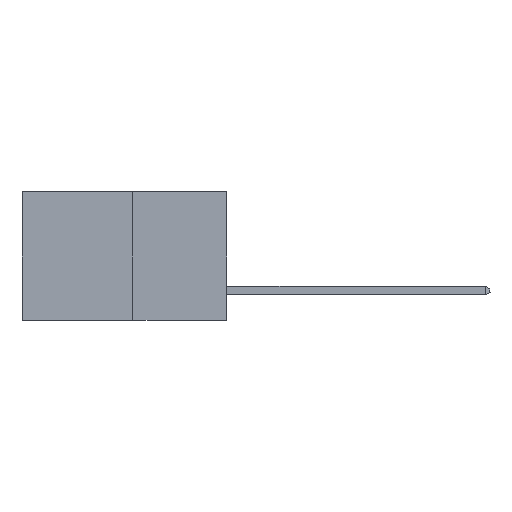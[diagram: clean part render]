
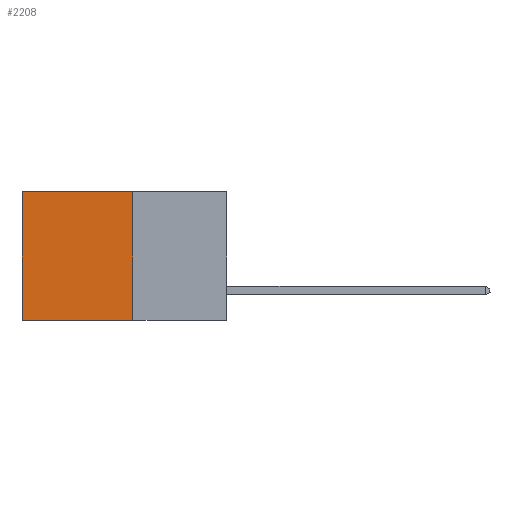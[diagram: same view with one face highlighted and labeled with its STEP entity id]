
A CAD part, left-side view. The second image highlights one B-rep face of the part: STEP entity #2208.
In plain terms, the highlighted planar face has unit normal (-1, 0, 0).
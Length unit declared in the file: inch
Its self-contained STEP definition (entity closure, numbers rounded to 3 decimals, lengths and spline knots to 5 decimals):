
#1157 = EDGE_CURVE ( 'NONE', #11840, #10073, #4215, .T. ) ;
#1207 = VECTOR ( 'NONE', #7720, 39.37008 ) ;
#1565 = EDGE_CURVE ( 'NONE', #10487, #11840, #7349, .T. ) ;
#2208 = ADVANCED_FACE ( 'NONE', ( #12992 ), #5448, .F. ) ;
#2436 = VECTOR ( 'NONE', #4837, 39.37008 ) ;
#4215 = LINE ( 'NONE', #14413, #1207 ) ;
#4347 = CARTESIAN_POINT ( 'NONE',  ( 0.277, 0.27, 0. ) ) ;
#4805 = CARTESIAN_POINT ( 'NONE',  ( 0.277, 0.27, -0.37 ) ) ;
#4837 = DIRECTION ( 'NONE',  ( 0., 1., 0. ) ) ;
#4951 = VECTOR ( 'NONE', #13122, 39.37008 ) ;
#5448 = PLANE ( 'NONE',  #10220 ) ;
#5536 = LINE ( 'NONE', #12847, #2436 ) ;
#5865 = VECTOR ( 'NONE', #13936, 39.37008 ) ;
#5984 = DIRECTION ( 'NONE',  ( 0., 0., -1. ) ) ;
#6015 = DIRECTION ( 'NONE',  ( 1., 0., 0. ) ) ;
#6047 = CARTESIAN_POINT ( 'NONE',  ( 0.277, 0.27, -0.37 ) ) ;
#6055 = VERTEX_POINT ( 'NONE', #6295 ) ;
#6295 = CARTESIAN_POINT ( 'NONE',  ( 0.277, 0.27, -0.37 ) ) ;
#7349 = LINE ( 'NONE', #13150, #4951 ) ;
#7720 = DIRECTION ( 'NONE',  ( 0., 0., -1. ) ) ;
#8882 = EDGE_CURVE ( 'NONE', #10487, #6055, #8899, .T. ) ;
#8899 = LINE ( 'NONE', #4805, #5865 ) ;
#9223 = ORIENTED_EDGE ( 'NONE', *, *, #1157, .T. ) ;
#9342 = ORIENTED_EDGE ( 'NONE', *, *, #11913, .F. ) ;
#9495 = ORIENTED_EDGE ( 'NONE', *, *, #8882, .F. ) ;
#9823 = ORIENTED_EDGE ( 'NONE', *, *, #1565, .T. ) ;
#10073 = VERTEX_POINT ( 'NONE', #14067 ) ;
#10220 = AXIS2_PLACEMENT_3D ( 'NONE', #6047, #6015, #5984 ) ;
#10487 = VERTEX_POINT ( 'NONE', #4347 ) ;
#11590 = CARTESIAN_POINT ( 'NONE',  ( 0.277, 0.59, 0. ) ) ;
#11840 = VERTEX_POINT ( 'NONE', #11590 ) ;
#11913 = EDGE_CURVE ( 'NONE', #6055, #10073, #5536, .T. ) ;
#12847 = CARTESIAN_POINT ( 'NONE',  ( 0.277, 0.27, -0.37 ) ) ;
#12992 = FACE_OUTER_BOUND ( 'NONE', #14480, .T. ) ;
#13122 = DIRECTION ( 'NONE',  ( 0., 1., 0. ) ) ;
#13150 = CARTESIAN_POINT ( 'NONE',  ( 0.277, 0.27, 0. ) ) ;
#13936 = DIRECTION ( 'NONE',  ( 0., 0., -1. ) ) ;
#14067 = CARTESIAN_POINT ( 'NONE',  ( 0.277, 0.59, -0.37 ) ) ;
#14413 = CARTESIAN_POINT ( 'NONE',  ( 0.277, 0.59, -0.37 ) ) ;
#14480 = EDGE_LOOP ( 'NONE', ( #9223, #9342, #9495, #9823 ) ) ;
